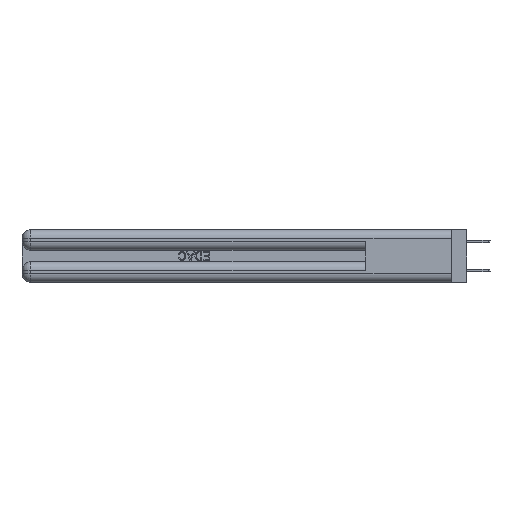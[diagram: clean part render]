
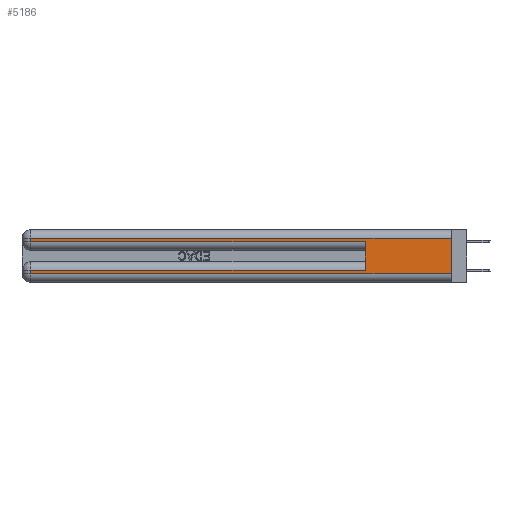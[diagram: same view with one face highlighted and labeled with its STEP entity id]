
A CAD part, left-side view. The second image highlights one B-rep face of the part: STEP entity #5186.
In plain terms, the highlighted planar face has unit normal (-1, 0, 0).
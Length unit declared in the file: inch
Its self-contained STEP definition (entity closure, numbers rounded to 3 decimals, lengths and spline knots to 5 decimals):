
#223 = CARTESIAN_POINT ( 'NONE',  ( 0., 0., 0.31 ) ) ;
#342 = VECTOR ( 'NONE', #33506, 39.37008 ) ;
#1695 = VERTEX_POINT ( 'NONE', #36663 ) ;
#2063 = CARTESIAN_POINT ( 'NONE',  ( 0., 0., 0.085 ) ) ;
#2112 = EDGE_LOOP ( 'NONE', ( #34839, #30516, #30704, #18634, #19118, #10534, #39868, #37213 ) ) ;
#2499 = EDGE_CURVE ( 'NONE', #36696, #23438, #33534, .T. ) ;
#4537 = CARTESIAN_POINT ( 'NONE',  ( 0., 0.6, 0.145 ) ) ;
#5165 = CARTESIAN_POINT ( 'NONE',  ( 0., 2.94, 0.31 ) ) ;
#5186 = ADVANCED_FACE ( 'NONE', ( #25769 ), #11828, .F. ) ;
#5384 = VECTOR ( 'NONE', #27882, 39.37008 ) ;
#5709 = EDGE_CURVE ( 'NONE', #16950, #1695, #11033, .T. ) ;
#7500 = EDGE_CURVE ( 'NONE', #23438, #22789, #39608, .T. ) ;
#7624 = DIRECTION ( 'NONE',  ( 0., 0., 1. ) ) ;
#7886 = DIRECTION ( 'NONE',  ( 0., -1., 0. ) ) ;
#8466 = DIRECTION ( 'NONE',  ( 0., 1., 0. ) ) ;
#9380 = LINE ( 'NONE', #31693, #342 ) ;
#9634 = VERTEX_POINT ( 'NONE', #18108 ) ;
#10212 = CARTESIAN_POINT ( 'NONE',  ( 0., 0., 0.06 ) ) ;
#10534 = ORIENTED_EDGE ( 'NONE', *, *, #5709, .T. ) ;
#11033 = LINE ( 'NONE', #2063, #38318 ) ;
#11773 = CARTESIAN_POINT ( 'NONE',  ( 0., 2.94, 0.37 ) ) ;
#11828 = PLANE ( 'NONE',  #29261 ) ;
#13049 = CARTESIAN_POINT ( 'NONE',  ( 0., 0., 0.31 ) ) ;
#15008 = EDGE_CURVE ( 'NONE', #36696, #22001, #9380, .T. ) ;
#15074 = DIRECTION ( 'NONE',  ( 0., 0., -1. ) ) ;
#15327 = EDGE_CURVE ( 'NONE', #22789, #40304, #40568, .T. ) ;
#16063 = CARTESIAN_POINT ( 'NONE',  ( 0., 2.94, 0.37 ) ) ;
#16950 = VERTEX_POINT ( 'NONE', #26328 ) ;
#17088 = LINE ( 'NONE', #16063, #26168 ) ;
#17384 = VECTOR ( 'NONE', #7624, 39.37008 ) ;
#18108 = CARTESIAN_POINT ( 'NONE',  ( 0., 2.94, 0.06 ) ) ;
#18634 = ORIENTED_EDGE ( 'NONE', *, *, #15327, .T. ) ;
#19118 = ORIENTED_EDGE ( 'NONE', *, *, #26889, .F. ) ;
#21363 = VECTOR ( 'NONE', #34102, 39.37008 ) ;
#22001 = VERTEX_POINT ( 'NONE', #10212 ) ;
#22789 = VERTEX_POINT ( 'NONE', #33405 ) ;
#23384 = LINE ( 'NONE', #39422, #21363 ) ;
#23438 = VERTEX_POINT ( 'NONE', #5165 ) ;
#24526 = DIRECTION ( 'NONE',  ( 1., 0., 0. ) ) ;
#24936 = VECTOR ( 'NONE', #35663, 39.37008 ) ;
#25507 = VECTOR ( 'NONE', #7886, 39.37008 ) ;
#25545 = LINE ( 'NONE', #4537, #17384 ) ;
#25769 = FACE_OUTER_BOUND ( 'NONE', #2112, .T. ) ;
#26126 = CARTESIAN_POINT ( 'NONE',  ( 0., 0.6, 0.285 ) ) ;
#26168 = VECTOR ( 'NONE', #29193, 39.37008 ) ;
#26328 = CARTESIAN_POINT ( 'NONE',  ( 0., 0.6, 0.085 ) ) ;
#26889 = EDGE_CURVE ( 'NONE', #16950, #40304, #25545, .T. ) ;
#27214 = CARTESIAN_POINT ( 'NONE',  ( 0., 0., 0.285 ) ) ;
#27882 = DIRECTION ( 'NONE',  ( 0., 0., -1. ) ) ;
#29193 = DIRECTION ( 'NONE',  ( 0., 0., -1. ) ) ;
#29261 = AXIS2_PLACEMENT_3D ( 'NONE', #34443, #24526, #15074 ) ;
#30516 = ORIENTED_EDGE ( 'NONE', *, *, #2499, .T. ) ;
#30704 = ORIENTED_EDGE ( 'NONE', *, *, #7500, .T. ) ;
#31693 = CARTESIAN_POINT ( 'NONE',  ( 0., 0., 0.37 ) ) ;
#33405 = CARTESIAN_POINT ( 'NONE',  ( 0., 2.94, 0.285 ) ) ;
#33506 = DIRECTION ( 'NONE',  ( 0., 0., -1. ) ) ;
#33534 = LINE ( 'NONE', #13049, #24936 ) ;
#34102 = DIRECTION ( 'NONE',  ( 0., -1., 0. ) ) ;
#34443 = CARTESIAN_POINT ( 'NONE',  ( 0., 0., 0.37 ) ) ;
#34839 = ORIENTED_EDGE ( 'NONE', *, *, #15008, .F. ) ;
#35387 = EDGE_CURVE ( 'NONE', #1695, #9634, #17088, .T. ) ;
#35663 = DIRECTION ( 'NONE',  ( 0., 1., 0. ) ) ;
#36663 = CARTESIAN_POINT ( 'NONE',  ( 0., 2.94, 0.085 ) ) ;
#36696 = VERTEX_POINT ( 'NONE', #223 ) ;
#37213 = ORIENTED_EDGE ( 'NONE', *, *, #38741, .T. ) ;
#38318 = VECTOR ( 'NONE', #8466, 39.37008 ) ;
#38741 = EDGE_CURVE ( 'NONE', #9634, #22001, #23384, .T. ) ;
#39422 = CARTESIAN_POINT ( 'NONE',  ( 0., 0., 0.06 ) ) ;
#39608 = LINE ( 'NONE', #11773, #5384 ) ;
#39868 = ORIENTED_EDGE ( 'NONE', *, *, #35387, .T. ) ;
#40304 = VERTEX_POINT ( 'NONE', #26126 ) ;
#40568 = LINE ( 'NONE', #27214, #25507 ) ;
